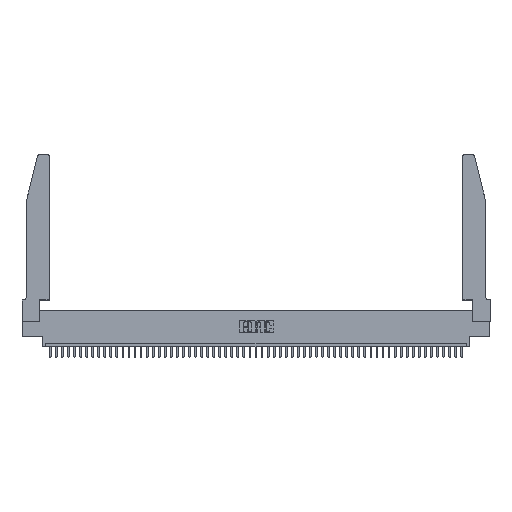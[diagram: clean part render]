
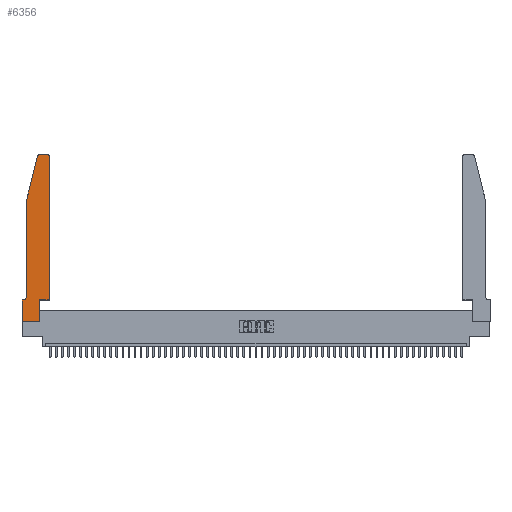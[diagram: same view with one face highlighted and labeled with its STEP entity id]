
A CAD part, top view. The second image highlights one B-rep face of the part: STEP entity #6356.
In plain terms, the highlighted planar face has unit normal (0, 0, 1).
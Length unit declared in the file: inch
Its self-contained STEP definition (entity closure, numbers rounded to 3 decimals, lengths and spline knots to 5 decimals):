
#392 = EDGE_CURVE ( 'NONE', #6359, #43778, #51588, .T. ) ;
#770 = VERTEX_POINT ( 'NONE', #20811 ) ;
#1056 = AXIS2_PLACEMENT_3D ( 'NONE', #16569, #32937, #28451 ) ;
#1099 = DIRECTION ( 'NONE',  ( -1., 0., 0. ) ) ;
#1256 = ORIENTED_EDGE ( 'NONE', *, *, #9184, .T. ) ;
#1391 = EDGE_CURVE ( 'NONE', #39617, #41044, #42385, .T. ) ;
#2579 = DIRECTION ( 'NONE',  ( 1., 0., 0. ) ) ;
#3505 = EDGE_CURVE ( 'NONE', #32561, #24181, #15106, .T. ) ;
#5100 = CARTESIAN_POINT ( 'NONE',  ( 0.25487, 2.72718, 0.37 ) ) ;
#6107 = AXIS2_PLACEMENT_3D ( 'NONE', #30803, #27169, #6150 ) ;
#6150 = DIRECTION ( 'NONE',  ( -1., 0., 0. ) ) ;
#6356 = ADVANCED_FACE ( 'NONE', ( #30801 ), #24807, .T. ) ;
#6359 = VERTEX_POINT ( 'NONE', #9877 ) ;
#8597 = ORIENTED_EDGE ( 'NONE', *, *, #51027, .T. ) ;
#8633 = LINE ( 'NONE', #17170, #51138 ) ;
#8641 = EDGE_CURVE ( 'NONE', #40149, #770, #45287, .T. ) ;
#8670 = VECTOR ( 'NONE', #49903, 39.37008 ) ;
#8759 = CARTESIAN_POINT ( 'NONE',  ( 0.4505, 0.35, 0.37 ) ) ;
#9184 = EDGE_CURVE ( 'NONE', #770, #30504, #20753, .T. ) ;
#9214 = CARTESIAN_POINT ( 'NONE',  ( 0., 0.35, 0.37 ) ) ;
#9877 = CARTESIAN_POINT ( 'NONE',  ( 0., 0., 0.37 ) ) ;
#10764 = VECTOR ( 'NONE', #52109, 39.37008 ) ;
#11236 = DIRECTION ( 'NONE',  ( -0.239, -0.971, 0. ) ) ;
#12067 = ORIENTED_EDGE ( 'NONE', *, *, #3505, .T. ) ;
#12293 = AXIS2_PLACEMENT_3D ( 'NONE', #41335, #50384, #17949 ) ;
#12553 = CARTESIAN_POINT ( 'NONE',  ( 0.284, 2.75, 0.37 ) ) ;
#13162 = CARTESIAN_POINT ( 'NONE',  ( 0.2865, 0.35, 0.37 ) ) ;
#13189 = DIRECTION ( 'NONE',  ( 1., 0., 0. ) ) ;
#13450 = ORIENTED_EDGE ( 'NONE', *, *, #8641, .T. ) ;
#14378 = EDGE_CURVE ( 'NONE', #21987, #20977, #48686, .T. ) ;
#14837 = CARTESIAN_POINT ( 'NONE',  ( 0.2605, 2.75, 0.37 ) ) ;
#15106 = LINE ( 'NONE', #21075, #8670 ) ;
#16221 = CARTESIAN_POINT ( 'NONE',  ( 0.2865, 0., 0.37 ) ) ;
#16470 = EDGE_LOOP ( 'NONE', ( #17927, #38223, #17694, #12067, #30516, #47606, #48462, #52670, #8597, #31240, #13450, #1256 ) ) ;
#16569 = CARTESIAN_POINT ( 'NONE',  ( 0.4205, 2.72, 0.37 ) ) ;
#16586 = CARTESIAN_POINT ( 'NONE',  ( 0., 0., 0.37 ) ) ;
#17160 = DIRECTION ( 'NONE',  ( 0., 1., 0. ) ) ;
#17170 = CARTESIAN_POINT ( 'NONE',  ( 0.4505, 0.35, 0.37 ) ) ;
#17244 = EDGE_CURVE ( 'NONE', #41044, #6359, #47381, .T. ) ;
#17694 = ORIENTED_EDGE ( 'NONE', *, *, #31164, .T. ) ;
#17766 = CARTESIAN_POINT ( 'NONE',  ( 0.0755, 0.35, 0.37 ) ) ;
#17927 = ORIENTED_EDGE ( 'NONE', *, *, #26867, .T. ) ;
#17949 = DIRECTION ( 'NONE',  ( 1., 0., 0. ) ) ;
#18918 = LINE ( 'NONE', #42988, #31180 ) ;
#20753 = CIRCLE ( 'NONE', #1056, 0.03 ) ;
#20773 = DIRECTION ( 'NONE',  ( 1., 0., 0. ) ) ;
#20811 = CARTESIAN_POINT ( 'NONE',  ( 0.4505, 2.72, 0.37 ) ) ;
#20977 = VERTEX_POINT ( 'NONE', #5100 ) ;
#21075 = CARTESIAN_POINT ( 'NONE',  ( 0.0755, 2., 0.37 ) ) ;
#21987 = VERTEX_POINT ( 'NONE', #12553 ) ;
#22694 = DIRECTION ( 'NONE',  ( 0., 0., 1. ) ) ;
#24181 = VERTEX_POINT ( 'NONE', #25661 ) ;
#24475 = CARTESIAN_POINT ( 'NONE',  ( 0.0755, 2., 0.37 ) ) ;
#24807 = PLANE ( 'NONE',  #12293 ) ;
#25262 = CARTESIAN_POINT ( 'NONE',  ( 0.4505, 0.35, 0.37 ) ) ;
#25463 = VECTOR ( 'NONE', #30602, 39.37008 ) ;
#25526 = EDGE_CURVE ( 'NONE', #24181, #39617, #30870, .T. ) ;
#25661 = CARTESIAN_POINT ( 'NONE',  ( 0.0755, 0.42, 0.37 ) ) ;
#25952 = VECTOR ( 'NONE', #11236, 39.37008 ) ;
#26867 = EDGE_CURVE ( 'NONE', #30504, #21987, #51350, .T. ) ;
#27169 = DIRECTION ( 'NONE',  ( 0., 0., -1. ) ) ;
#28451 = DIRECTION ( 'NONE',  ( 1., 0., 0. ) ) ;
#30504 = VERTEX_POINT ( 'NONE', #35721 ) ;
#30516 = ORIENTED_EDGE ( 'NONE', *, *, #25526, .T. ) ;
#30602 = DIRECTION ( 'NONE',  ( 0., -1., 0. ) ) ;
#30801 = FACE_OUTER_BOUND ( 'NONE', #16470, .T. ) ;
#30803 = CARTESIAN_POINT ( 'NONE',  ( 0.0055, 0.42, 0.37 ) ) ;
#30870 = CIRCLE ( 'NONE', #6107, 0.07 ) ;
#31163 = LINE ( 'NONE', #35302, #25952 ) ;
#31164 = EDGE_CURVE ( 'NONE', #20977, #32561, #31163, .T. ) ;
#31180 = VECTOR ( 'NONE', #51322, 39.37008 ) ;
#31240 = ORIENTED_EDGE ( 'NONE', *, *, #44603, .T. ) ;
#32561 = VERTEX_POINT ( 'NONE', #24475 ) ;
#32717 = VERTEX_POINT ( 'NONE', #13162 ) ;
#32937 = DIRECTION ( 'NONE',  ( 0., 0., 1. ) ) ;
#34368 = AXIS2_PLACEMENT_3D ( 'NONE', #35107, #22694, #2579 ) ;
#35107 = CARTESIAN_POINT ( 'NONE',  ( 0.284, 2.72, 0.37 ) ) ;
#35302 = CARTESIAN_POINT ( 'NONE',  ( 0.0755, 2., 0.37 ) ) ;
#35418 = VECTOR ( 'NONE', #13189, 39.37008 ) ;
#35721 = CARTESIAN_POINT ( 'NONE',  ( 0.4205, 2.75, 0.37 ) ) ;
#38223 = ORIENTED_EDGE ( 'NONE', *, *, #14378, .T. ) ;
#39617 = VERTEX_POINT ( 'NONE', #45046 ) ;
#40149 = VERTEX_POINT ( 'NONE', #8759 ) ;
#41044 = VERTEX_POINT ( 'NONE', #9214 ) ;
#41335 = CARTESIAN_POINT ( 'NONE',  ( 0., 0.35, 0.37 ) ) ;
#41748 = CARTESIAN_POINT ( 'NONE',  ( 0., 0., 0.37 ) ) ;
#42385 = LINE ( 'NONE', #17766, #48206 ) ;
#42988 = CARTESIAN_POINT ( 'NONE',  ( 0.2865, 0.35, 0.37 ) ) ;
#43778 = VERTEX_POINT ( 'NONE', #16221 ) ;
#44603 = EDGE_CURVE ( 'NONE', #32717, #40149, #8633, .T. ) ;
#45046 = CARTESIAN_POINT ( 'NONE',  ( 0.0055, 0.35, 0.37 ) ) ;
#45287 = LINE ( 'NONE', #25262, #50497 ) ;
#47381 = LINE ( 'NONE', #41748, #25463 ) ;
#47606 = ORIENTED_EDGE ( 'NONE', *, *, #1391, .T. ) ;
#48206 = VECTOR ( 'NONE', #1099, 39.37008 ) ;
#48462 = ORIENTED_EDGE ( 'NONE', *, *, #17244, .T. ) ;
#48686 = CIRCLE ( 'NONE', #34368, 0.03 ) ;
#49903 = DIRECTION ( 'NONE',  ( 0., -1., 0. ) ) ;
#50384 = DIRECTION ( 'NONE',  ( 0., 0., 1. ) ) ;
#50497 = VECTOR ( 'NONE', #17160, 39.37008 ) ;
#51027 = EDGE_CURVE ( 'NONE', #43778, #32717, #18918, .T. ) ;
#51138 = VECTOR ( 'NONE', #20773, 39.37008 ) ;
#51322 = DIRECTION ( 'NONE',  ( 0., 1., 0. ) ) ;
#51350 = LINE ( 'NONE', #14837, #10764 ) ;
#51588 = LINE ( 'NONE', #16586, #35418 ) ;
#52109 = DIRECTION ( 'NONE',  ( -1., 0., 0. ) ) ;
#52670 = ORIENTED_EDGE ( 'NONE', *, *, #392, .T. ) ;
